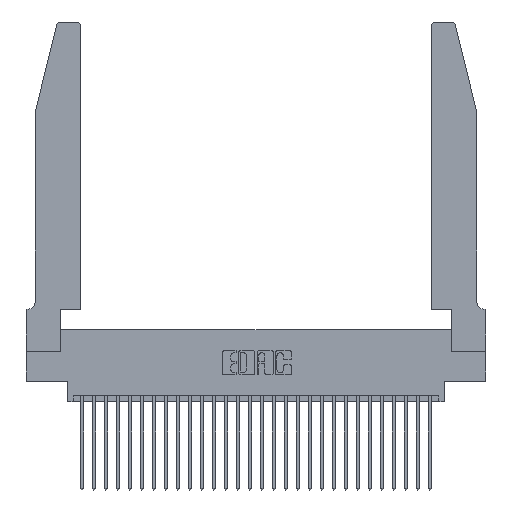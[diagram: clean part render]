
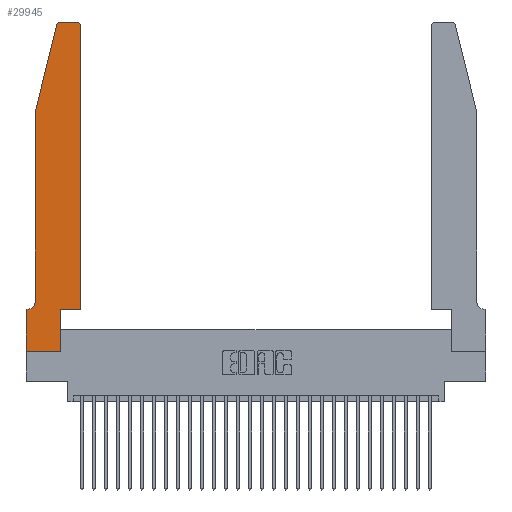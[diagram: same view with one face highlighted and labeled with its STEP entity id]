
A CAD part, top view. The second image highlights one B-rep face of the part: STEP entity #29945.
In plain terms, the highlighted planar face has unit normal (0, 0, 1).
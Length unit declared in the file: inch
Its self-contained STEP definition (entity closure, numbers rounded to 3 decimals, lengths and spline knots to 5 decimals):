
#180 = VERTEX_POINT ( 'NONE', #8905 ) ;
#207 = ORIENTED_EDGE ( 'NONE', *, *, #28402, .T. ) ;
#816 = DIRECTION ( 'NONE',  ( 0., 1., 0. ) ) ;
#919 = EDGE_CURVE ( 'NONE', #3102, #28542, #10909, .T. ) ;
#1306 = DIRECTION ( 'NONE',  ( -1., 0., 0. ) ) ;
#1646 = CARTESIAN_POINT ( 'NONE',  ( 0., 0.35, 0.37 ) ) ;
#2568 = CARTESIAN_POINT ( 'NONE',  ( 0.4505, 0.35, 0.37 ) ) ;
#2768 = ORIENTED_EDGE ( 'NONE', *, *, #22911, .T. ) ;
#2874 = DIRECTION ( 'NONE',  ( -0.239, -0.971, 0. ) ) ;
#3102 = VERTEX_POINT ( 'NONE', #4722 ) ;
#3343 = ORIENTED_EDGE ( 'NONE', *, *, #919, .T. ) ;
#3449 = AXIS2_PLACEMENT_3D ( 'NONE', #28369, #5023, #7335 ) ;
#3549 = DIRECTION ( 'NONE',  ( 0., 0., -1. ) ) ;
#3984 = VECTOR ( 'NONE', #7682, 39.37008 ) ;
#4068 = EDGE_CURVE ( 'NONE', #13766, #26018, #19851, .T. ) ;
#4123 = CARTESIAN_POINT ( 'NONE',  ( 0.4505, 2.72, 0.37 ) ) ;
#4722 = CARTESIAN_POINT ( 'NONE',  ( 0.4205, 2.75, 0.37 ) ) ;
#5023 = DIRECTION ( 'NONE',  ( 0., 0., 1. ) ) ;
#5085 = CARTESIAN_POINT ( 'NONE',  ( 0.0055, 0.35, 0.37 ) ) ;
#5166 = CARTESIAN_POINT ( 'NONE',  ( 0.0755, 0.35, 0.37 ) ) ;
#5626 = ORIENTED_EDGE ( 'NONE', *, *, #11170, .T. ) ;
#5664 = VECTOR ( 'NONE', #816, 39.37008 ) ;
#5756 = VERTEX_POINT ( 'NONE', #11544 ) ;
#6447 = DIRECTION ( 'NONE',  ( 1., 0., 0. ) ) ;
#6930 = CARTESIAN_POINT ( 'NONE',  ( 0.2865, 0., 0.37 ) ) ;
#7156 = CARTESIAN_POINT ( 'NONE',  ( 0.4505, 0.35, 0.37 ) ) ;
#7211 = VECTOR ( 'NONE', #9333, 39.37008 ) ;
#7267 = VERTEX_POINT ( 'NONE', #6930 ) ;
#7335 = DIRECTION ( 'NONE',  ( 1., 0., 0. ) ) ;
#7682 = DIRECTION ( 'NONE',  ( -1., 0., 0. ) ) ;
#8001 = DIRECTION ( 'NONE',  ( 0., 0., 1. ) ) ;
#8234 = DIRECTION ( 'NONE',  ( 0., -1., 0. ) ) ;
#8257 = VECTOR ( 'NONE', #6447, 39.37008 ) ;
#8439 = CIRCLE ( 'NONE', #3449, 0.03 ) ;
#8784 = LINE ( 'NONE', #5166, #22273 ) ;
#8801 = VERTEX_POINT ( 'NONE', #21127 ) ;
#8867 = EDGE_CURVE ( 'NONE', #180, #16888, #27938, .T. ) ;
#8905 = CARTESIAN_POINT ( 'NONE',  ( 0.0755, 0.42, 0.37 ) ) ;
#9142 = VECTOR ( 'NONE', #21008, 39.37008 ) ;
#9333 = DIRECTION ( 'NONE',  ( 0., 1., 0. ) ) ;
#9393 = ORIENTED_EDGE ( 'NONE', *, *, #4068, .T. ) ;
#10317 = CIRCLE ( 'NONE', #24471, 0.03 ) ;
#10498 = CARTESIAN_POINT ( 'NONE',  ( 0.0055, 0.42, 0.37 ) ) ;
#10670 = DIRECTION ( 'NONE',  ( 1., 0., 0. ) ) ;
#10828 = VERTEX_POINT ( 'NONE', #26720 ) ;
#10909 = LINE ( 'NONE', #26121, #3984 ) ;
#11052 = ORIENTED_EDGE ( 'NONE', *, *, #28564, .T. ) ;
#11170 = EDGE_CURVE ( 'NONE', #7267, #13766, #24272, .T. ) ;
#11390 = VECTOR ( 'NONE', #8234, 39.37008 ) ;
#11544 = CARTESIAN_POINT ( 'NONE',  ( 0., 0.35, 0.37 ) ) ;
#11790 = AXIS2_PLACEMENT_3D ( 'NONE', #10498, #3549, #1306 ) ;
#12251 = CARTESIAN_POINT ( 'NONE',  ( 0.2865, 0.35, 0.37 ) ) ;
#12623 = VERTEX_POINT ( 'NONE', #4123 ) ;
#12661 = EDGE_CURVE ( 'NONE', #20010, #8801, #23213, .T. ) ;
#13342 = CARTESIAN_POINT ( 'NONE',  ( 0.25487, 2.72718, 0.37 ) ) ;
#13766 = VERTEX_POINT ( 'NONE', #19932 ) ;
#14149 = ORIENTED_EDGE ( 'NONE', *, *, #8867, .T. ) ;
#14774 = AXIS2_PLACEMENT_3D ( 'NONE', #1646, #29362, #20516 ) ;
#15192 = CARTESIAN_POINT ( 'NONE',  ( 0., 0., 0.37 ) ) ;
#15305 = EDGE_CURVE ( 'NONE', #5756, #10828, #24502, .T. ) ;
#16601 = VECTOR ( 'NONE', #17708, 39.37008 ) ;
#16888 = VERTEX_POINT ( 'NONE', #5085 ) ;
#17708 = DIRECTION ( 'NONE',  ( 1., 0., 0. ) ) ;
#17907 = LINE ( 'NONE', #18664, #9142 ) ;
#18291 = CARTESIAN_POINT ( 'NONE',  ( 0., 0., 0.37 ) ) ;
#18664 = CARTESIAN_POINT ( 'NONE',  ( 0.0755, 2., 0.37 ) ) ;
#18952 = CARTESIAN_POINT ( 'NONE',  ( 0.284, 2.75, 0.37 ) ) ;
#19628 = LINE ( 'NONE', #2568, #7211 ) ;
#19851 = LINE ( 'NONE', #20267, #16601 ) ;
#19932 = CARTESIAN_POINT ( 'NONE',  ( 0.2865, 0.35, 0.37 ) ) ;
#20010 = VERTEX_POINT ( 'NONE', #13342 ) ;
#20159 = EDGE_CURVE ( 'NONE', #12623, #3102, #8439, .T. ) ;
#20267 = CARTESIAN_POINT ( 'NONE',  ( 0.4505, 0.35, 0.37 ) ) ;
#20516 = DIRECTION ( 'NONE',  ( 1., 0., 0. ) ) ;
#21008 = DIRECTION ( 'NONE',  ( 0., -1., 0. ) ) ;
#21109 = FACE_OUTER_BOUND ( 'NONE', #29685, .T. ) ;
#21127 = CARTESIAN_POINT ( 'NONE',  ( 0.0755, 2., 0.37 ) ) ;
#22273 = VECTOR ( 'NONE', #23739, 39.37008 ) ;
#22346 = ORIENTED_EDGE ( 'NONE', *, *, #15305, .T. ) ;
#22911 = EDGE_CURVE ( 'NONE', #10828, #7267, #25751, .T. ) ;
#23213 = LINE ( 'NONE', #28364, #27489 ) ;
#23739 = DIRECTION ( 'NONE',  ( -1., 0., 0. ) ) ;
#24272 = LINE ( 'NONE', #12251, #5664 ) ;
#24465 = ORIENTED_EDGE ( 'NONE', *, *, #12661, .T. ) ;
#24471 = AXIS2_PLACEMENT_3D ( 'NONE', #29097, #8001, #10670 ) ;
#24502 = LINE ( 'NONE', #15192, #11390 ) ;
#24864 = PLANE ( 'NONE',  #14774 ) ;
#24883 = ORIENTED_EDGE ( 'NONE', *, *, #29558, .T. ) ;
#25751 = LINE ( 'NONE', #18291, #8257 ) ;
#25771 = ORIENTED_EDGE ( 'NONE', *, *, #20159, .T. ) ;
#26018 = VERTEX_POINT ( 'NONE', #7156 ) ;
#26121 = CARTESIAN_POINT ( 'NONE',  ( 0.2605, 2.75, 0.37 ) ) ;
#26720 = CARTESIAN_POINT ( 'NONE',  ( 0., 0., 0.37 ) ) ;
#27489 = VECTOR ( 'NONE', #2874, 39.37008 ) ;
#27544 = EDGE_CURVE ( 'NONE', #28542, #20010, #10317, .T. ) ;
#27938 = CIRCLE ( 'NONE', #11790, 0.07 ) ;
#28364 = CARTESIAN_POINT ( 'NONE',  ( 0.0755, 2., 0.37 ) ) ;
#28369 = CARTESIAN_POINT ( 'NONE',  ( 0.4205, 2.72, 0.37 ) ) ;
#28402 = EDGE_CURVE ( 'NONE', #8801, #180, #17907, .T. ) ;
#28542 = VERTEX_POINT ( 'NONE', #18952 ) ;
#28564 = EDGE_CURVE ( 'NONE', #16888, #5756, #8784, .T. ) ;
#29097 = CARTESIAN_POINT ( 'NONE',  ( 0.284, 2.72, 0.37 ) ) ;
#29362 = DIRECTION ( 'NONE',  ( 0., 0., 1. ) ) ;
#29558 = EDGE_CURVE ( 'NONE', #26018, #12623, #19628, .T. ) ;
#29685 = EDGE_LOOP ( 'NONE', ( #3343, #29870, #24465, #207, #14149, #11052, #22346, #2768, #5626, #9393, #24883, #25771 ) ) ;
#29870 = ORIENTED_EDGE ( 'NONE', *, *, #27544, .T. ) ;
#29945 = ADVANCED_FACE ( 'NONE', ( #21109 ), #24864, .T. ) ;
